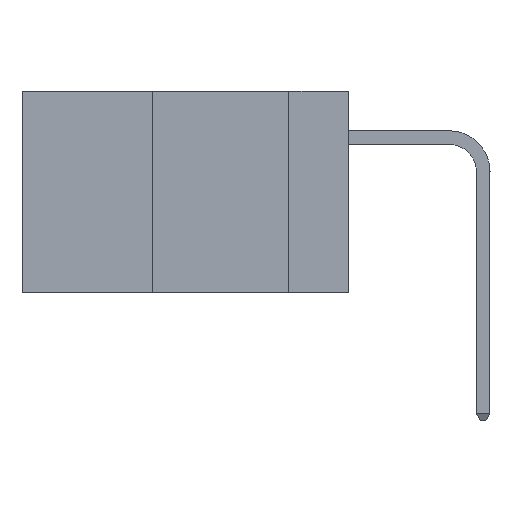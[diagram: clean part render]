
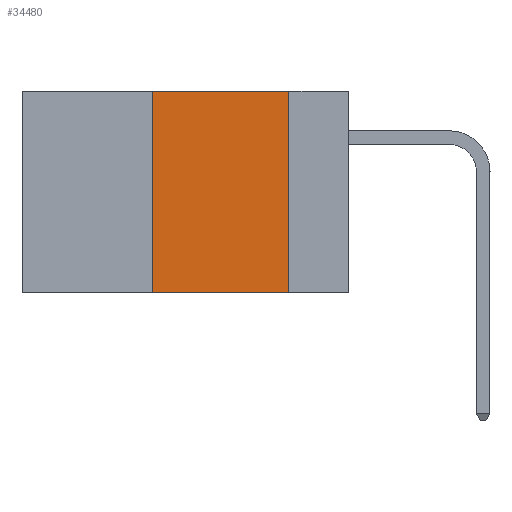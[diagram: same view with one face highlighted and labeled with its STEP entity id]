
A CAD part, left-side view. The second image highlights one B-rep face of the part: STEP entity #34480.
In plain terms, the highlighted planar face has unit normal (-1, 0, 0).
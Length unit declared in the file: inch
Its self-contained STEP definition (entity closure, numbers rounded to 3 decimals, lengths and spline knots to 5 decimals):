
#1715 = LINE ( 'NONE', #17476, #23559 ) ;
#2005 = DIRECTION ( 'NONE',  ( 1., 0., 0. ) ) ;
#2180 = PLANE ( 'NONE',  #37033 ) ;
#2366 = DIRECTION ( 'NONE',  ( 0., -1., 0. ) ) ;
#3888 = VECTOR ( 'NONE', #2366, 39.37008 ) ;
#5288 = FACE_OUTER_BOUND ( 'NONE', #21138, .T. ) ;
#6874 = ORIENTED_EDGE ( 'NONE', *, *, #47777, .T. ) ;
#8105 = EDGE_CURVE ( 'NONE', #37945, #29679, #27851, .T. ) ;
#9965 = CARTESIAN_POINT ( 'NONE',  ( 0., 0.6, 0. ) ) ;
#11159 = LINE ( 'NONE', #34751, #40372 ) ;
#11768 = ORIENTED_EDGE ( 'NONE', *, *, #8105, .F. ) ;
#12716 = EDGE_CURVE ( 'NONE', #29679, #39941, #35438, .T. ) ;
#13337 = ORIENTED_EDGE ( 'NONE', *, *, #16137, .F. ) ;
#15238 = CARTESIAN_POINT ( 'NONE',  ( 0., 0.11, 0. ) ) ;
#16137 = EDGE_CURVE ( 'NONE', #39941, #26390, #1715, .T. ) ;
#16677 = CARTESIAN_POINT ( 'NONE',  ( 0., 0.36, 0. ) ) ;
#17476 = CARTESIAN_POINT ( 'NONE',  ( 0., 0.11, 0. ) ) ;
#20301 = CARTESIAN_POINT ( 'NONE',  ( 0., 0.11, -0.37 ) ) ;
#21138 = EDGE_LOOP ( 'NONE', ( #13337, #27085, #11768, #6874 ) ) ;
#22369 = CARTESIAN_POINT ( 'NONE',  ( 0., 0.6, 0. ) ) ;
#23559 = VECTOR ( 'NONE', #48715, 39.37008 ) ;
#25403 = CARTESIAN_POINT ( 'NONE',  ( 0., 0.36, 0. ) ) ;
#25736 = DIRECTION ( 'NONE',  ( 0., 0., -1. ) ) ;
#26390 = VERTEX_POINT ( 'NONE', #20301 ) ;
#27085 = ORIENTED_EDGE ( 'NONE', *, *, #12716, .F. ) ;
#27851 = LINE ( 'NONE', #25403, #40048 ) ;
#29679 = VERTEX_POINT ( 'NONE', #16677 ) ;
#34480 = ADVANCED_FACE ( 'NONE', ( #5288 ), #2180, .F. ) ;
#34751 = CARTESIAN_POINT ( 'NONE',  ( 0., 0.6, -0.37 ) ) ;
#35438 = LINE ( 'NONE', #22369, #3888 ) ;
#37033 = AXIS2_PLACEMENT_3D ( 'NONE', #9965, #2005, #25736 ) ;
#37945 = VERTEX_POINT ( 'NONE', #50214 ) ;
#39941 = VERTEX_POINT ( 'NONE', #15238 ) ;
#40048 = VECTOR ( 'NONE', #48850, 39.37008 ) ;
#40372 = VECTOR ( 'NONE', #50034, 39.37008 ) ;
#47777 = EDGE_CURVE ( 'NONE', #37945, #26390, #11159, .T. ) ;
#48715 = DIRECTION ( 'NONE',  ( 0., 0., -1. ) ) ;
#48850 = DIRECTION ( 'NONE',  ( 0., 0., 1. ) ) ;
#50034 = DIRECTION ( 'NONE',  ( 0., -1., 0. ) ) ;
#50214 = CARTESIAN_POINT ( 'NONE',  ( 0., 0.36, -0.37 ) ) ;
